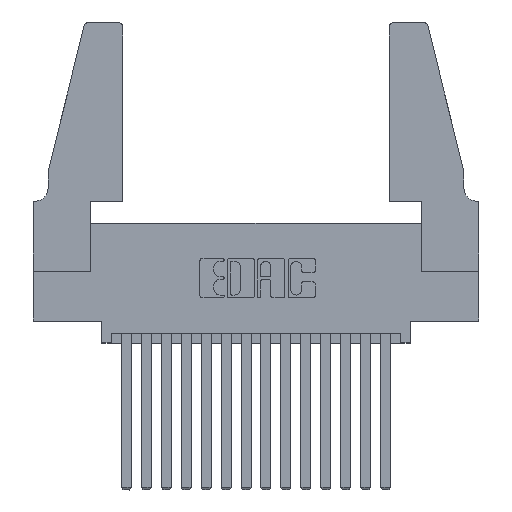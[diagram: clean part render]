
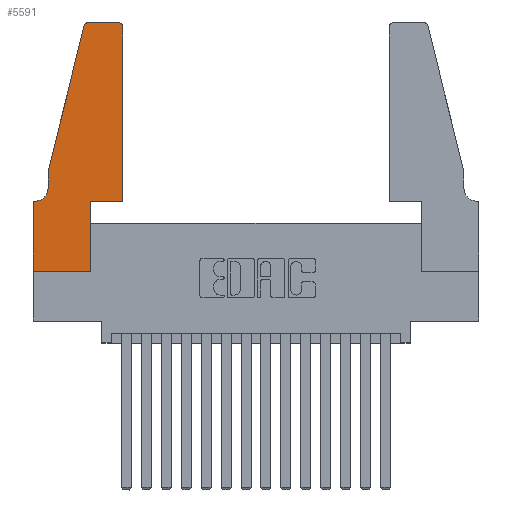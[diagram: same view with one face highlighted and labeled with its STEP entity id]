
A CAD part, top view. The second image highlights one B-rep face of the part: STEP entity #5591.
In plain terms, the highlighted planar face has unit normal (0, 0, 1).
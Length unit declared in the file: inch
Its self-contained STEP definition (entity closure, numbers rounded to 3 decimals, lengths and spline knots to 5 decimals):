
#62 = CARTESIAN_POINT ( 'NONE',  ( 0., 0.35, 0.37 ) ) ;
#224 = AXIS2_PLACEMENT_3D ( 'NONE', #6659, #4056, #4119 ) ;
#404 = VERTEX_POINT ( 'NONE', #15535 ) ;
#426 = EDGE_CURVE ( 'NONE', #7748, #3802, #11960, .T. ) ;
#660 = CARTESIAN_POINT ( 'NONE',  ( 0., 0.35, 0.37 ) ) ;
#707 = CARTESIAN_POINT ( 'NONE',  ( 0., 0., 0.37 ) ) ;
#720 = VECTOR ( 'NONE', #7181, 39.37008 ) ;
#765 = CARTESIAN_POINT ( 'NONE',  ( 0.0755, 0.5, 0.37 ) ) ;
#813 = VECTOR ( 'NONE', #16597, 39.37008 ) ;
#1040 = ORIENTED_EDGE ( 'NONE', *, *, #11751, .T. ) ;
#1064 = CARTESIAN_POINT ( 'NONE',  ( 0.0755, 0.35, 0.37 ) ) ;
#1442 = EDGE_LOOP ( 'NONE', ( #4738, #6093, #16088, #10255, #5151, #6624, #1040, #8343, #15461, #3719, #13037, #8728 ) ) ;
#1621 = AXIS2_PLACEMENT_3D ( 'NONE', #12240, #16111, #5869 ) ;
#1938 = CARTESIAN_POINT ( 'NONE',  ( 0.2865, 0.35, 0.37 ) ) ;
#2080 = VERTEX_POINT ( 'NONE', #8311 ) ;
#2142 = LINE ( 'NONE', #1938, #720 ) ;
#2270 = DIRECTION ( 'NONE',  ( 0., 1., 0. ) ) ;
#2292 = CARTESIAN_POINT ( 'NONE',  ( 0.2865, 0.35, 0.37 ) ) ;
#2369 = DIRECTION ( 'NONE',  ( -1., 0., 0. ) ) ;
#2642 = CARTESIAN_POINT ( 'NONE',  ( 0.284, 1.22, 0.37 ) ) ;
#2914 = EDGE_CURVE ( 'NONE', #4640, #2080, #15576, .T. ) ;
#3032 = VERTEX_POINT ( 'NONE', #765 ) ;
#3054 = VERTEX_POINT ( 'NONE', #9779 ) ;
#3279 = DIRECTION ( 'NONE',  ( 1., 0., 0. ) ) ;
#3468 = VERTEX_POINT ( 'NONE', #16506 ) ;
#3569 = CARTESIAN_POINT ( 'NONE',  ( 0.0755, 0.5, 0.37 ) ) ;
#3656 = AXIS2_PLACEMENT_3D ( 'NONE', #2642, #5260, #5380 ) ;
#3719 = ORIENTED_EDGE ( 'NONE', *, *, #2914, .T. ) ;
#3802 = VERTEX_POINT ( 'NONE', #4832 ) ;
#3990 = VECTOR ( 'NONE', #4179, 39.37008 ) ;
#4056 = DIRECTION ( 'NONE',  ( 0., 0., -1. ) ) ;
#4057 = VECTOR ( 'NONE', #2369, 39.37008 ) ;
#4119 = DIRECTION ( 'NONE',  ( -1., 0., 0. ) ) ;
#4135 = EDGE_CURVE ( 'NONE', #3032, #3468, #6489, .T. ) ;
#4169 = EDGE_CURVE ( 'NONE', #12161, #11847, #10182, .T. ) ;
#4179 = DIRECTION ( 'NONE',  ( -0.239, -0.971, 0. ) ) ;
#4640 = VERTEX_POINT ( 'NONE', #2292 ) ;
#4738 = ORIENTED_EDGE ( 'NONE', *, *, #7483, .T. ) ;
#4832 = CARTESIAN_POINT ( 'NONE',  ( 0.2865, 0., 0.37 ) ) ;
#5151 = ORIENTED_EDGE ( 'NONE', *, *, #13810, .T. ) ;
#5260 = DIRECTION ( 'NONE',  ( 0., 0., 1. ) ) ;
#5380 = DIRECTION ( 'NONE',  ( 1., 0., 0. ) ) ;
#5591 = ADVANCED_FACE ( 'NONE', ( #10576 ), #14776, .T. ) ;
#5667 = DIRECTION ( 'NONE',  ( 1., 0., 0. ) ) ;
#5676 = VECTOR ( 'NONE', #6461, 39.37008 ) ;
#5803 = CARTESIAN_POINT ( 'NONE',  ( 0.2605, 1.25, 0.37 ) ) ;
#5869 = DIRECTION ( 'NONE',  ( 1., 0., 0. ) ) ;
#6093 = ORIENTED_EDGE ( 'NONE', *, *, #7055, .T. ) ;
#6229 = LINE ( 'NONE', #14440, #3990 ) ;
#6461 = DIRECTION ( 'NONE',  ( 1., 0., 0. ) ) ;
#6489 = LINE ( 'NONE', #3569, #813 ) ;
#6624 = ORIENTED_EDGE ( 'NONE', *, *, #4169, .T. ) ;
#6659 = CARTESIAN_POINT ( 'NONE',  ( 0.0055, 0.42, 0.37 ) ) ;
#7055 = EDGE_CURVE ( 'NONE', #15527, #404, #14988, .T. ) ;
#7107 = DIRECTION ( 'NONE',  ( -1., 0., 0. ) ) ;
#7181 = DIRECTION ( 'NONE',  ( 0., 1., 0. ) ) ;
#7483 = EDGE_CURVE ( 'NONE', #13389, #15527, #15991, .T. ) ;
#7596 = CARTESIAN_POINT ( 'NONE',  ( 0.284, 1.25, 0.37 ) ) ;
#7661 = CIRCLE ( 'NONE', #224, 0.07 ) ;
#7748 = VERTEX_POINT ( 'NONE', #7949 ) ;
#7949 = CARTESIAN_POINT ( 'NONE',  ( 0., 0., 0.37 ) ) ;
#8203 = EDGE_CURVE ( 'NONE', #404, #3032, #6229, .T. ) ;
#8311 = CARTESIAN_POINT ( 'NONE',  ( 0.4505, 0.35, 0.37 ) ) ;
#8343 = ORIENTED_EDGE ( 'NONE', *, *, #426, .T. ) ;
#8662 = VECTOR ( 'NONE', #7107, 39.37008 ) ;
#8728 = ORIENTED_EDGE ( 'NONE', *, *, #12345, .T. ) ;
#9369 = CIRCLE ( 'NONE', #1621, 0.03 ) ;
#9779 = CARTESIAN_POINT ( 'NONE',  ( 0.4505, 1.22, 0.37 ) ) ;
#9881 = EDGE_CURVE ( 'NONE', #2080, #3054, #13450, .T. ) ;
#10000 = DIRECTION ( 'NONE',  ( 0., -1., 0. ) ) ;
#10182 = LINE ( 'NONE', #1064, #4057 ) ;
#10255 = ORIENTED_EDGE ( 'NONE', *, *, #4135, .T. ) ;
#10529 = CARTESIAN_POINT ( 'NONE',  ( 0., 0., 0.37 ) ) ;
#10576 = FACE_OUTER_BOUND ( 'NONE', #1442, .T. ) ;
#11086 = DIRECTION ( 'NONE',  ( 0., 0., 1. ) ) ;
#11567 = VECTOR ( 'NONE', #10000, 39.37008 ) ;
#11751 = EDGE_CURVE ( 'NONE', #11847, #7748, #14458, .T. ) ;
#11847 = VERTEX_POINT ( 'NONE', #62 ) ;
#11960 = LINE ( 'NONE', #10529, #5676 ) ;
#12161 = VERTEX_POINT ( 'NONE', #14688 ) ;
#12240 = CARTESIAN_POINT ( 'NONE',  ( 0.4205, 1.22, 0.37 ) ) ;
#12345 = EDGE_CURVE ( 'NONE', #3054, #13389, #9369, .T. ) ;
#12912 = VECTOR ( 'NONE', #5667, 39.37008 ) ;
#13037 = ORIENTED_EDGE ( 'NONE', *, *, #9881, .T. ) ;
#13389 = VERTEX_POINT ( 'NONE', #14773 ) ;
#13450 = LINE ( 'NONE', #13995, #15700 ) ;
#13810 = EDGE_CURVE ( 'NONE', #3468, #12161, #7661, .T. ) ;
#13995 = CARTESIAN_POINT ( 'NONE',  ( 0.4505, 0.35, 0.37 ) ) ;
#14440 = CARTESIAN_POINT ( 'NONE',  ( 0.0755, 0.5, 0.37 ) ) ;
#14458 = LINE ( 'NONE', #707, #11567 ) ;
#14688 = CARTESIAN_POINT ( 'NONE',  ( 0.0055, 0.35, 0.37 ) ) ;
#14740 = EDGE_CURVE ( 'NONE', #3802, #4640, #2142, .T. ) ;
#14773 = CARTESIAN_POINT ( 'NONE',  ( 0.4205, 1.25, 0.37 ) ) ;
#14775 = CARTESIAN_POINT ( 'NONE',  ( 0.4505, 0.35, 0.37 ) ) ;
#14776 = PLANE ( 'NONE',  #16292 ) ;
#14988 = CIRCLE ( 'NONE', #3656, 0.03 ) ;
#15461 = ORIENTED_EDGE ( 'NONE', *, *, #14740, .T. ) ;
#15527 = VERTEX_POINT ( 'NONE', #7596 ) ;
#15535 = CARTESIAN_POINT ( 'NONE',  ( 0.25487, 1.22718, 0.37 ) ) ;
#15576 = LINE ( 'NONE', #14775, #12912 ) ;
#15700 = VECTOR ( 'NONE', #2270, 39.37008 ) ;
#15991 = LINE ( 'NONE', #5803, #8662 ) ;
#16088 = ORIENTED_EDGE ( 'NONE', *, *, #8203, .T. ) ;
#16111 = DIRECTION ( 'NONE',  ( 0., 0., 1. ) ) ;
#16292 = AXIS2_PLACEMENT_3D ( 'NONE', #660, #11086, #3279 ) ;
#16506 = CARTESIAN_POINT ( 'NONE',  ( 0.0755, 0.42, 0.37 ) ) ;
#16597 = DIRECTION ( 'NONE',  ( 0., -1., 0. ) ) ;
